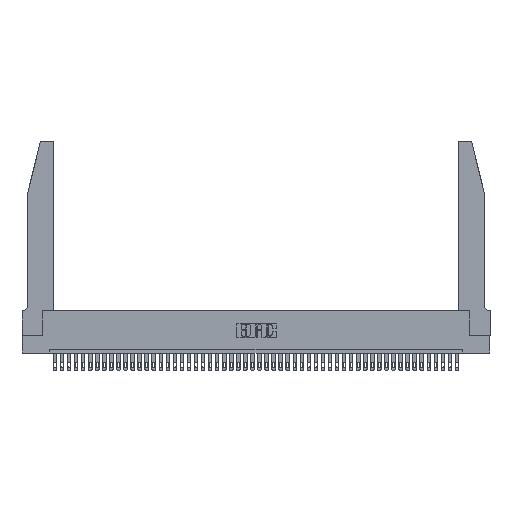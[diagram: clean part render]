
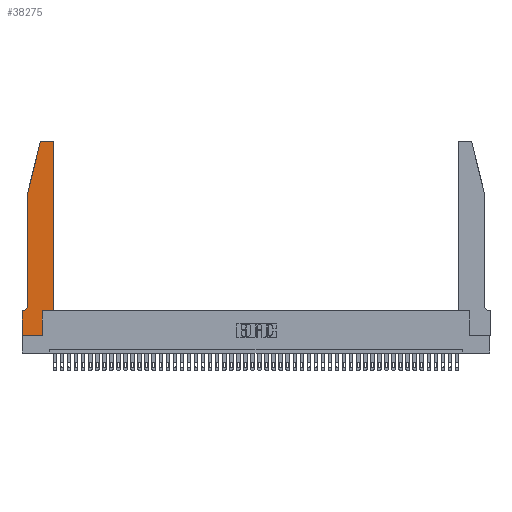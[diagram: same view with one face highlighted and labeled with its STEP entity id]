
A CAD part, top view. The second image highlights one B-rep face of the part: STEP entity #38275.
In plain terms, the highlighted planar face has unit normal (0, 0, 1).
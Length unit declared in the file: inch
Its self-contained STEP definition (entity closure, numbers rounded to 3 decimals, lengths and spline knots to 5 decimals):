
#398 = CARTESIAN_POINT ( 'NONE',  ( 0.2605, 2.75, 0.37 ) ) ;
#1277 = EDGE_CURVE ( 'NONE', #9104, #17927, #36092, .T. ) ;
#1435 = LINE ( 'NONE', #29985, #10908 ) ;
#2587 = ORIENTED_EDGE ( 'NONE', *, *, #6085, .T. ) ;
#3103 = VERTEX_POINT ( 'NONE', #16814 ) ;
#3260 = CARTESIAN_POINT ( 'NONE',  ( 0.0755, 0.42, 0.37 ) ) ;
#3453 = VERTEX_POINT ( 'NONE', #3260 ) ;
#4230 = CARTESIAN_POINT ( 'NONE',  ( 0.2865, 0., 0.37 ) ) ;
#5267 = CARTESIAN_POINT ( 'NONE',  ( 0.4505, 0.35, 0.37 ) ) ;
#5409 = ORIENTED_EDGE ( 'NONE', *, *, #26947, .T. ) ;
#6085 = EDGE_CURVE ( 'NONE', #13328, #35706, #44617, .T. ) ;
#6367 = CARTESIAN_POINT ( 'NONE',  ( 0.4205, 2.75, 0.37 ) ) ;
#6464 = VECTOR ( 'NONE', #31401, 39.37008 ) ;
#7161 = DIRECTION ( 'NONE',  ( 1., 0., 0. ) ) ;
#7329 = CARTESIAN_POINT ( 'NONE',  ( 0.284, 2.72, 0.37 ) ) ;
#7626 = ORIENTED_EDGE ( 'NONE', *, *, #41488, .T. ) ;
#8031 = VECTOR ( 'NONE', #11764, 39.37008 ) ;
#9104 = VERTEX_POINT ( 'NONE', #41898 ) ;
#9483 = FACE_OUTER_BOUND ( 'NONE', #33387, .T. ) ;
#9594 = AXIS2_PLACEMENT_3D ( 'NONE', #19455, #16005, #38559 ) ;
#10160 = DIRECTION ( 'NONE',  ( -1., 0., 0. ) ) ;
#10326 = ORIENTED_EDGE ( 'NONE', *, *, #44112, .T. ) ;
#10373 = ORIENTED_EDGE ( 'NONE', *, *, #32081, .T. ) ;
#10409 = CARTESIAN_POINT ( 'NONE',  ( 0.4205, 2.72, 0.37 ) ) ;
#10908 = VECTOR ( 'NONE', #15427, 39.37008 ) ;
#11764 = DIRECTION ( 'NONE',  ( -0.239, -0.971, 0. ) ) ;
#12089 = ORIENTED_EDGE ( 'NONE', *, *, #40481, .T. ) ;
#12112 = CARTESIAN_POINT ( 'NONE',  ( 0., 0., 0.37 ) ) ;
#12564 = EDGE_CURVE ( 'NONE', #28798, #9104, #1435, .T. ) ;
#13247 = DIRECTION ( 'NONE',  ( 0., 0., 1. ) ) ;
#13328 = VERTEX_POINT ( 'NONE', #41937 ) ;
#13395 = VERTEX_POINT ( 'NONE', #27271 ) ;
#13518 = CARTESIAN_POINT ( 'NONE',  ( 0., 0.35, 0.37 ) ) ;
#13612 = LINE ( 'NONE', #22218, #8031 ) ;
#13790 = VECTOR ( 'NONE', #44807, 39.37008 ) ;
#15427 = DIRECTION ( 'NONE',  ( 0., 1., 0. ) ) ;
#16005 = DIRECTION ( 'NONE',  ( 0., 0., -1. ) ) ;
#16814 = CARTESIAN_POINT ( 'NONE',  ( 0.284, 2.75, 0.37 ) ) ;
#17036 = CARTESIAN_POINT ( 'NONE',  ( 0.2865, 0.35, 0.37 ) ) ;
#17560 = DIRECTION ( 'NONE',  ( 0., 0., 1. ) ) ;
#17927 = VERTEX_POINT ( 'NONE', #6367 ) ;
#18154 = LINE ( 'NONE', #17036, #6464 ) ;
#19157 = ORIENTED_EDGE ( 'NONE', *, *, #26653, .T. ) ;
#19209 = DIRECTION ( 'NONE',  ( 1., 0., 0. ) ) ;
#19455 = CARTESIAN_POINT ( 'NONE',  ( 0.0055, 0.42, 0.37 ) ) ;
#19884 = CARTESIAN_POINT ( 'NONE',  ( 0., 0., 0.37 ) ) ;
#20541 = VERTEX_POINT ( 'NONE', #24740 ) ;
#22218 = CARTESIAN_POINT ( 'NONE',  ( 0.0755, 2., 0.37 ) ) ;
#23245 = CARTESIAN_POINT ( 'NONE',  ( 0.0755, 2., 0.37 ) ) ;
#23298 = LINE ( 'NONE', #19884, #13790 ) ;
#23399 = DIRECTION ( 'NONE',  ( 0., -1., 0. ) ) ;
#23407 = VERTEX_POINT ( 'NONE', #4230 ) ;
#23480 = EDGE_CURVE ( 'NONE', #17927, #3103, #38852, .T. ) ;
#23629 = EDGE_CURVE ( 'NONE', #32574, #3453, #33322, .T. ) ;
#23704 = AXIS2_PLACEMENT_3D ( 'NONE', #34586, #13247, #7161 ) ;
#24740 = CARTESIAN_POINT ( 'NONE',  ( 0.25487, 2.72718, 0.37 ) ) ;
#24939 = DIRECTION ( 'NONE',  ( 1., 0., 0. ) ) ;
#25080 = ORIENTED_EDGE ( 'NONE', *, *, #23480, .T. ) ;
#25128 = VECTOR ( 'NONE', #19209, 39.37008 ) ;
#26538 = ORIENTED_EDGE ( 'NONE', *, *, #23629, .T. ) ;
#26553 = CIRCLE ( 'NONE', #39038, 0.03 ) ;
#26653 = EDGE_CURVE ( 'NONE', #33536, #23407, #32015, .T. ) ;
#26947 = EDGE_CURVE ( 'NONE', #3453, #13328, #43065, .T. ) ;
#27271 = CARTESIAN_POINT ( 'NONE',  ( 0.2865, 0.35, 0.37 ) ) ;
#27333 = PLANE ( 'NONE',  #23704 ) ;
#28798 = VERTEX_POINT ( 'NONE', #5267 ) ;
#29985 = CARTESIAN_POINT ( 'NONE',  ( 0.4505, 0.35, 0.37 ) ) ;
#31401 = DIRECTION ( 'NONE',  ( 0., 1., 0. ) ) ;
#31681 = VECTOR ( 'NONE', #10160, 39.37008 ) ;
#32015 = LINE ( 'NONE', #12112, #40292 ) ;
#32081 = EDGE_CURVE ( 'NONE', #23407, #13395, #18154, .T. ) ;
#32181 = CARTESIAN_POINT ( 'NONE',  ( 0., 0., 0.37 ) ) ;
#32574 = VERTEX_POINT ( 'NONE', #37840 ) ;
#33024 = DIRECTION ( 'NONE',  ( 1., 0., 0. ) ) ;
#33322 = LINE ( 'NONE', #23245, #38322 ) ;
#33387 = EDGE_LOOP ( 'NONE', ( #25080, #7626, #36936, #26538, #5409, #2587, #12089, #19157, #10373, #10326, #42658, #35214 ) ) ;
#33536 = VERTEX_POINT ( 'NONE', #32181 ) ;
#33812 = CARTESIAN_POINT ( 'NONE',  ( 0.0755, 0.35, 0.37 ) ) ;
#34586 = CARTESIAN_POINT ( 'NONE',  ( 0., 0.35, 0.37 ) ) ;
#35156 = VECTOR ( 'NONE', #40466, 39.37008 ) ;
#35214 = ORIENTED_EDGE ( 'NONE', *, *, #1277, .T. ) ;
#35706 = VERTEX_POINT ( 'NONE', #13518 ) ;
#35980 = DIRECTION ( 'NONE',  ( 0., 0., 1. ) ) ;
#35989 = EDGE_CURVE ( 'NONE', #20541, #32574, #13612, .T. ) ;
#36092 = CIRCLE ( 'NONE', #39011, 0.03 ) ;
#36936 = ORIENTED_EDGE ( 'NONE', *, *, #35989, .T. ) ;
#37840 = CARTESIAN_POINT ( 'NONE',  ( 0.0755, 2., 0.37 ) ) ;
#38275 = ADVANCED_FACE ( 'NONE', ( #9483 ), #27333, .T. ) ;
#38322 = VECTOR ( 'NONE', #23399, 39.37008 ) ;
#38559 = DIRECTION ( 'NONE',  ( -1., 0., 0. ) ) ;
#38852 = LINE ( 'NONE', #398, #31681 ) ;
#39011 = AXIS2_PLACEMENT_3D ( 'NONE', #10409, #17560, #39459 ) ;
#39038 = AXIS2_PLACEMENT_3D ( 'NONE', #7329, #35980, #24939 ) ;
#39459 = DIRECTION ( 'NONE',  ( 1., 0., 0. ) ) ;
#40292 = VECTOR ( 'NONE', #33024, 39.37008 ) ;
#40466 = DIRECTION ( 'NONE',  ( -1., 0., 0. ) ) ;
#40481 = EDGE_CURVE ( 'NONE', #35706, #33536, #23298, .T. ) ;
#41488 = EDGE_CURVE ( 'NONE', #3103, #20541, #26553, .T. ) ;
#41809 = LINE ( 'NONE', #43797, #25128 ) ;
#41898 = CARTESIAN_POINT ( 'NONE',  ( 0.4505, 2.72, 0.37 ) ) ;
#41937 = CARTESIAN_POINT ( 'NONE',  ( 0.0055, 0.35, 0.37 ) ) ;
#42658 = ORIENTED_EDGE ( 'NONE', *, *, #12564, .T. ) ;
#43065 = CIRCLE ( 'NONE', #9594, 0.07 ) ;
#43797 = CARTESIAN_POINT ( 'NONE',  ( 0.4505, 0.35, 0.37 ) ) ;
#44112 = EDGE_CURVE ( 'NONE', #13395, #28798, #41809, .T. ) ;
#44617 = LINE ( 'NONE', #33812, #35156 ) ;
#44807 = DIRECTION ( 'NONE',  ( 0., -1., 0. ) ) ;
